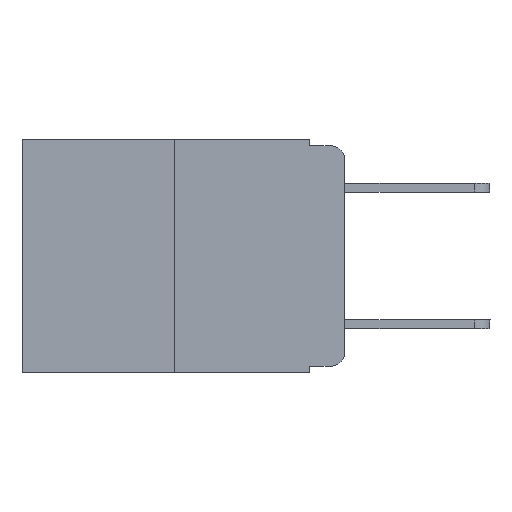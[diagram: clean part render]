
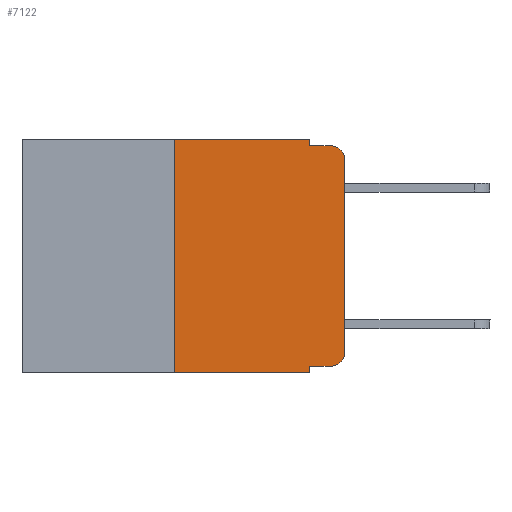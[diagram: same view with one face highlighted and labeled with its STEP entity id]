
A CAD part, left-side view. The second image highlights one B-rep face of the part: STEP entity #7122.
In plain terms, the highlighted planar face has unit normal (-1, 0, 0).
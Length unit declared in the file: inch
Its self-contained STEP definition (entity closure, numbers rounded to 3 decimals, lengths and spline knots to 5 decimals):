
#437 = VECTOR ( 'NONE', #7491, 39.37008 ) ;
#743 = VERTEX_POINT ( 'NONE', #1069 ) ;
#948 = VECTOR ( 'NONE', #8896, 39.37008 ) ;
#963 = DIRECTION ( 'NONE',  ( 0., -1., 0. ) ) ;
#970 = CARTESIAN_POINT ( 'NONE',  ( 0., 0.051, -0.343 ) ) ;
#1069 = CARTESIAN_POINT ( 'NONE',  ( 0., 0.02, -0.333 ) ) ;
#1304 = VECTOR ( 'NONE', #20001, 39.37008 ) ;
#1347 = AXIS2_PLACEMENT_3D ( 'NONE', #20087, #3616, #11907 ) ;
#2438 = CARTESIAN_POINT ( 'NONE',  ( 0., 0.051, 0. ) ) ;
#2762 = LINE ( 'NONE', #21037, #16689 ) ;
#2994 = VERTEX_POINT ( 'NONE', #20304 ) ;
#3198 = CARTESIAN_POINT ( 'NONE',  ( 0., 0.02, -0.313 ) ) ;
#3526 = FACE_OUTER_BOUND ( 'NONE', #18698, .T. ) ;
#3616 = DIRECTION ( 'NONE',  ( 1., 0., 0. ) ) ;
#4059 = ORIENTED_EDGE ( 'NONE', *, *, #15732, .T. ) ;
#4408 = ORIENTED_EDGE ( 'NONE', *, *, #8995, .F. ) ;
#4636 = CARTESIAN_POINT ( 'NONE',  ( 0., 0., -0.313 ) ) ;
#4948 = ORIENTED_EDGE ( 'NONE', *, *, #17805, .T. ) ;
#5447 = AXIS2_PLACEMENT_3D ( 'NONE', #3198, #16922, #10367 ) ;
#5487 = EDGE_CURVE ( 'NONE', #9323, #13061, #20585, .T. ) ;
#5718 = VECTOR ( 'NONE', #14682, 39.37008 ) ;
#5764 = EDGE_CURVE ( 'NONE', #9128, #10879, #11704, .T. ) ;
#5962 = CARTESIAN_POINT ( 'NONE',  ( 0., 0.051, 0. ) ) ;
#6008 = ORIENTED_EDGE ( 'NONE', *, *, #5487, .F. ) ;
#7122 = ADVANCED_FACE ( 'NONE', ( #3526 ), #8385, .F. ) ;
#7396 = CARTESIAN_POINT ( 'NONE',  ( 0., 0., 0. ) ) ;
#7491 = DIRECTION ( 'NONE',  ( 0., 0., 1. ) ) ;
#7507 = VECTOR ( 'NONE', #19720, 39.37008 ) ;
#7889 = CARTESIAN_POINT ( 'NONE',  ( 0., 0.25, -0.343 ) ) ;
#8014 = CARTESIAN_POINT ( 'NONE',  ( 0., 0.051, 0. ) ) ;
#8287 = CIRCLE ( 'NONE', #8407, 0.02 ) ;
#8305 = CARTESIAN_POINT ( 'NONE',  ( 0., 0.051, -0.333 ) ) ;
#8385 = PLANE ( 'NONE',  #1347 ) ;
#8407 = AXIS2_PLACEMENT_3D ( 'NONE', #16628, #9660, #11414 ) ;
#8829 = EDGE_CURVE ( 'NONE', #2994, #21314, #8287, .T. ) ;
#8896 = DIRECTION ( 'NONE',  ( 0., 0., -1. ) ) ;
#8992 = EDGE_CURVE ( 'NONE', #11848, #9128, #2762, .T. ) ;
#8995 = EDGE_CURVE ( 'NONE', #10879, #21314, #17209, .T. ) ;
#9128 = VERTEX_POINT ( 'NONE', #5962 ) ;
#9159 = DIRECTION ( 'NONE',  ( 0., 0., 1. ) ) ;
#9323 = VERTEX_POINT ( 'NONE', #8305 ) ;
#9524 = ORIENTED_EDGE ( 'NONE', *, *, #8992, .F. ) ;
#9660 = DIRECTION ( 'NONE',  ( -1., 0., 0. ) ) ;
#10271 = ORIENTED_EDGE ( 'NONE', *, *, #16857, .T. ) ;
#10367 = DIRECTION ( 'NONE',  ( 0., 0., -1. ) ) ;
#10497 = LINE ( 'NONE', #18431, #1304 ) ;
#10655 = VERTEX_POINT ( 'NONE', #7889 ) ;
#10879 = VERTEX_POINT ( 'NONE', #12736 ) ;
#11106 = CARTESIAN_POINT ( 'NONE',  ( 0., 0.051, -0.01 ) ) ;
#11414 = DIRECTION ( 'NONE',  ( 0., 0., -1. ) ) ;
#11688 = LINE ( 'NONE', #7396, #20063 ) ;
#11704 = LINE ( 'NONE', #8014, #7507 ) ;
#11848 = VERTEX_POINT ( 'NONE', #19565 ) ;
#11907 = DIRECTION ( 'NONE',  ( 0., 0., -1. ) ) ;
#11946 = CARTESIAN_POINT ( 'NONE',  ( 0., 0.02, -0.01 ) ) ;
#12736 = CARTESIAN_POINT ( 'NONE',  ( 0., 0.051, -0.01 ) ) ;
#13061 = VERTEX_POINT ( 'NONE', #970 ) ;
#13808 = CARTESIAN_POINT ( 'NONE',  ( 0., 0.25, 0. ) ) ;
#14061 = EDGE_CURVE ( 'NONE', #9323, #743, #10497, .T. ) ;
#14607 = CIRCLE ( 'NONE', #5447, 0.02 ) ;
#14682 = DIRECTION ( 'NONE',  ( 0., -1., 0. ) ) ;
#15681 = LINE ( 'NONE', #16451, #5718 ) ;
#15732 = EDGE_CURVE ( 'NONE', #10655, #13061, #15681, .T. ) ;
#15923 = LINE ( 'NONE', #13808, #437 ) ;
#16451 = CARTESIAN_POINT ( 'NONE',  ( 0., 0.473, -0.343 ) ) ;
#16628 = CARTESIAN_POINT ( 'NONE',  ( 0., 0.02, -0.03 ) ) ;
#16689 = VECTOR ( 'NONE', #963, 39.37008 ) ;
#16857 = EDGE_CURVE ( 'NONE', #743, #17351, #14607, .T. ) ;
#16922 = DIRECTION ( 'NONE',  ( -1., 0., 0. ) ) ;
#17143 = EDGE_CURVE ( 'NONE', #10655, #11848, #15923, .T. ) ;
#17209 = LINE ( 'NONE', #11106, #21072 ) ;
#17351 = VERTEX_POINT ( 'NONE', #4636 ) ;
#17805 = EDGE_CURVE ( 'NONE', #17351, #2994, #11688, .T. ) ;
#17885 = ORIENTED_EDGE ( 'NONE', *, *, #8829, .T. ) ;
#17944 = DIRECTION ( 'NONE',  ( 0., -1., 0. ) ) ;
#18431 = CARTESIAN_POINT ( 'NONE',  ( 0., 0.051, -0.333 ) ) ;
#18667 = ORIENTED_EDGE ( 'NONE', *, *, #5764, .F. ) ;
#18698 = EDGE_LOOP ( 'NONE', ( #4948, #17885, #4408, #18667, #9524, #21041, #4059, #6008, #20948, #10271 ) ) ;
#19565 = CARTESIAN_POINT ( 'NONE',  ( 0., 0.25, 0. ) ) ;
#19720 = DIRECTION ( 'NONE',  ( 0., 0., -1. ) ) ;
#20001 = DIRECTION ( 'NONE',  ( 0., -1., 0. ) ) ;
#20063 = VECTOR ( 'NONE', #9159, 39.37008 ) ;
#20087 = CARTESIAN_POINT ( 'NONE',  ( 0., 0.473, 0. ) ) ;
#20304 = CARTESIAN_POINT ( 'NONE',  ( 0., 0., -0.03 ) ) ;
#20585 = LINE ( 'NONE', #2438, #948 ) ;
#20948 = ORIENTED_EDGE ( 'NONE', *, *, #14061, .T. ) ;
#21037 = CARTESIAN_POINT ( 'NONE',  ( 0., 0.473, 0. ) ) ;
#21041 = ORIENTED_EDGE ( 'NONE', *, *, #17143, .F. ) ;
#21072 = VECTOR ( 'NONE', #17944, 39.37008 ) ;
#21314 = VERTEX_POINT ( 'NONE', #11946 ) ;
